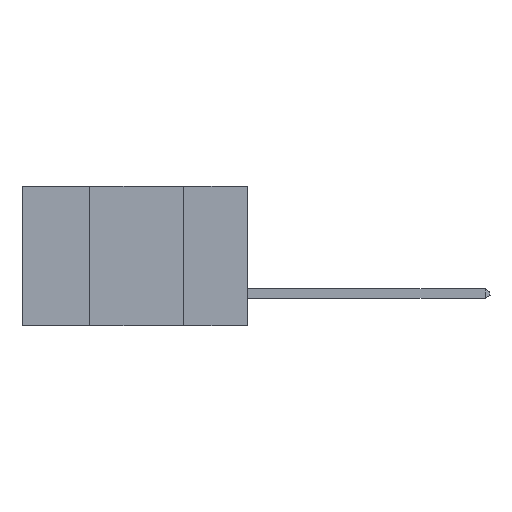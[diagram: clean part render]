
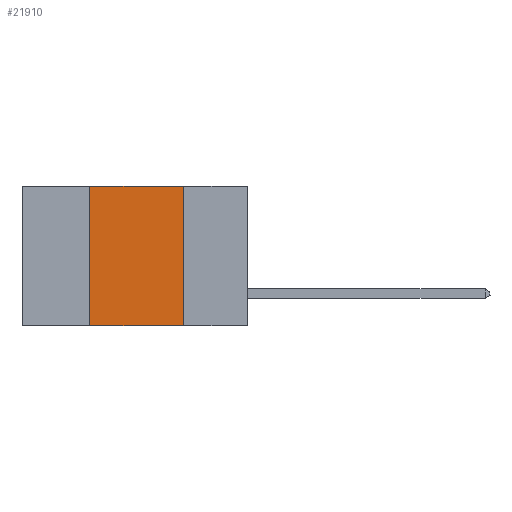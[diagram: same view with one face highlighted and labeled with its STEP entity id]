
A CAD part, left-side view. The second image highlights one B-rep face of the part: STEP entity #21910.
In plain terms, the highlighted planar face has unit normal (-1, 0, 0).
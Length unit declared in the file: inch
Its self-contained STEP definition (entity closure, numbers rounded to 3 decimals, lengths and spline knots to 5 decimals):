
#904 = VECTOR ( 'NONE', #11754, 39.37008 ) ;
#1652 = VECTOR ( 'NONE', #18349, 39.37008 ) ;
#1691 = CARTESIAN_POINT ( 'NONE',  ( 0., 0.17, 0. ) ) ;
#1760 = VERTEX_POINT ( 'NONE', #11583 ) ;
#1801 = VERTEX_POINT ( 'NONE', #13297 ) ;
#2445 = CARTESIAN_POINT ( 'NONE',  ( 0., 0.6, 0. ) ) ;
#3332 = CARTESIAN_POINT ( 'NONE',  ( 0., 0.6, 0. ) ) ;
#3619 = PLANE ( 'NONE',  #5303 ) ;
#4501 = EDGE_CURVE ( 'NONE', #1801, #18138, #8438, .T. ) ;
#5303 = AXIS2_PLACEMENT_3D ( 'NONE', #3332, #10504, #17050 ) ;
#5526 = ORIENTED_EDGE ( 'NONE', *, *, #16691, .T. ) ;
#5747 = ORIENTED_EDGE ( 'NONE', *, *, #20070, .F. ) ;
#7547 = FACE_OUTER_BOUND ( 'NONE', #15728, .T. ) ;
#8154 = CARTESIAN_POINT ( 'NONE',  ( 0., 0.6, -0.37 ) ) ;
#8438 = LINE ( 'NONE', #2445, #15931 ) ;
#10000 = CARTESIAN_POINT ( 'NONE',  ( 0., 0.17, 0. ) ) ;
#10356 = LINE ( 'NONE', #20710, #18943 ) ;
#10504 = DIRECTION ( 'NONE',  ( 1., 0., 0. ) ) ;
#11099 = VERTEX_POINT ( 'NONE', #12446 ) ;
#11583 = CARTESIAN_POINT ( 'NONE',  ( 0., 0.42, -0.37 ) ) ;
#11754 = DIRECTION ( 'NONE',  ( 0., 0., -1. ) ) ;
#11873 = LINE ( 'NONE', #8154, #1652 ) ;
#12446 = CARTESIAN_POINT ( 'NONE',  ( 0., 0.17, -0.37 ) ) ;
#13297 = CARTESIAN_POINT ( 'NONE',  ( 0., 0.42, 0. ) ) ;
#13426 = ORIENTED_EDGE ( 'NONE', *, *, #4501, .F. ) ;
#15728 = EDGE_LOOP ( 'NONE', ( #20117, #13426, #5747, #5526 ) ) ;
#15931 = VECTOR ( 'NONE', #19622, 39.37008 ) ;
#16691 = EDGE_CURVE ( 'NONE', #1760, #11099, #11873, .T. ) ;
#17050 = DIRECTION ( 'NONE',  ( 0., 0., -1. ) ) ;
#17694 = DIRECTION ( 'NONE',  ( 0., 0., 1. ) ) ;
#18138 = VERTEX_POINT ( 'NONE', #1691 ) ;
#18349 = DIRECTION ( 'NONE',  ( 0., -1., 0. ) ) ;
#18943 = VECTOR ( 'NONE', #17694, 39.37008 ) ;
#19127 = LINE ( 'NONE', #10000, #904 ) ;
#19622 = DIRECTION ( 'NONE',  ( 0., -1., 0. ) ) ;
#20070 = EDGE_CURVE ( 'NONE', #1760, #1801, #10356, .T. ) ;
#20117 = ORIENTED_EDGE ( 'NONE', *, *, #21093, .F. ) ;
#20710 = CARTESIAN_POINT ( 'NONE',  ( 0., 0.42, 0. ) ) ;
#21093 = EDGE_CURVE ( 'NONE', #18138, #11099, #19127, .T. ) ;
#21910 = ADVANCED_FACE ( 'NONE', ( #7547 ), #3619, .F. ) ;
